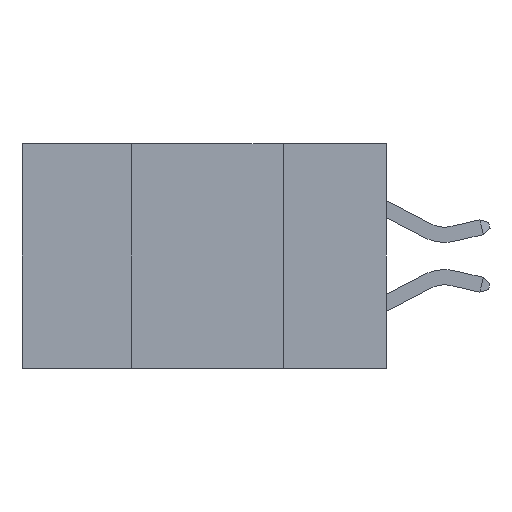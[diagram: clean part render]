
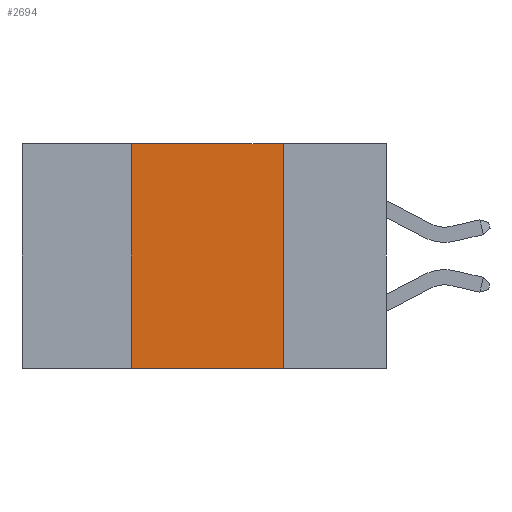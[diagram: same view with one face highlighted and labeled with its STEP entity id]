
A CAD part, left-side view. The second image highlights one B-rep face of the part: STEP entity #2694.
In plain terms, the highlighted planar face has unit normal (-1, 0, 0).
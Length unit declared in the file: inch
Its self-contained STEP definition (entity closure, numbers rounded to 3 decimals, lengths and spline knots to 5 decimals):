
#6 = ORIENTED_EDGE ( 'NONE', *, *, #6930, .F. ) ;
#354 = EDGE_CURVE ( 'NONE', #3824, #7180, #7502, .T. ) ;
#509 = VECTOR ( 'NONE', #660, 39.37008 ) ;
#660 = DIRECTION ( 'NONE',  ( 0., -1., 0. ) ) ;
#751 = LINE ( 'NONE', #3225, #9808 ) ;
#1506 = DIRECTION ( 'NONE',  ( 0., 0., -1. ) ) ;
#1706 = VECTOR ( 'NONE', #2016, 39.37008 ) ;
#2016 = DIRECTION ( 'NONE',  ( 0., -1., 0. ) ) ;
#2683 = VERTEX_POINT ( 'NONE', #4203 ) ;
#2694 = ADVANCED_FACE ( 'NONE', ( #7635 ), #3492, .F. ) ;
#2878 = DIRECTION ( 'NONE',  ( 1., 0., 0. ) ) ;
#3049 = EDGE_CURVE ( 'NONE', #9948, #2683, #7104, .T. ) ;
#3120 = LINE ( 'NONE', #5588, #8806 ) ;
#3216 = ORIENTED_EDGE ( 'NONE', *, *, #7131, .F. ) ;
#3225 = CARTESIAN_POINT ( 'NONE',  ( 0., 0.42, -0.37 ) ) ;
#3415 = AXIS2_PLACEMENT_3D ( 'NONE', #6662, #2878, #5106 ) ;
#3492 = PLANE ( 'NONE',  #3415 ) ;
#3824 = VERTEX_POINT ( 'NONE', #4612 ) ;
#4082 = DIRECTION ( 'NONE',  ( 0., 0., 1. ) ) ;
#4203 = CARTESIAN_POINT ( 'NONE',  ( 0., 0.17, -0.37 ) ) ;
#4612 = CARTESIAN_POINT ( 'NONE',  ( 0., 0.42, 0. ) ) ;
#5106 = DIRECTION ( 'NONE',  ( 0., 0., -1. ) ) ;
#5588 = CARTESIAN_POINT ( 'NONE',  ( 0., 0.17, -0.37 ) ) ;
#6408 = CARTESIAN_POINT ( 'NONE',  ( 0., 0.6, -0.37 ) ) ;
#6662 = CARTESIAN_POINT ( 'NONE',  ( 0., 0.6, 0. ) ) ;
#6842 = CARTESIAN_POINT ( 'NONE',  ( 0., 0.6, 0. ) ) ;
#6930 = EDGE_CURVE ( 'NONE', #7180, #2683, #3120, .T. ) ;
#7104 = LINE ( 'NONE', #6408, #509 ) ;
#7131 = EDGE_CURVE ( 'NONE', #9948, #3824, #751, .T. ) ;
#7160 = CARTESIAN_POINT ( 'NONE',  ( 0., 0.42, -0.37 ) ) ;
#7180 = VERTEX_POINT ( 'NONE', #9287 ) ;
#7502 = LINE ( 'NONE', #6842, #1706 ) ;
#7635 = FACE_OUTER_BOUND ( 'NONE', #9999, .T. ) ;
#7944 = ORIENTED_EDGE ( 'NONE', *, *, #3049, .T. ) ;
#7954 = ORIENTED_EDGE ( 'NONE', *, *, #354, .F. ) ;
#8806 = VECTOR ( 'NONE', #1506, 39.37008 ) ;
#9287 = CARTESIAN_POINT ( 'NONE',  ( 0., 0.17, 0. ) ) ;
#9808 = VECTOR ( 'NONE', #4082, 39.37008 ) ;
#9948 = VERTEX_POINT ( 'NONE', #7160 ) ;
#9999 = EDGE_LOOP ( 'NONE', ( #6, #7954, #3216, #7944 ) ) ;
